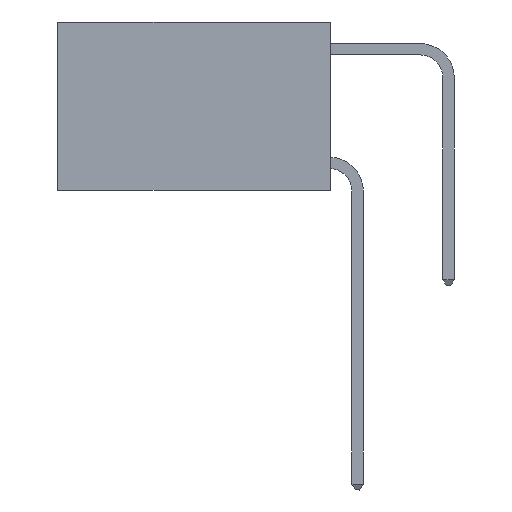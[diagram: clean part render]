
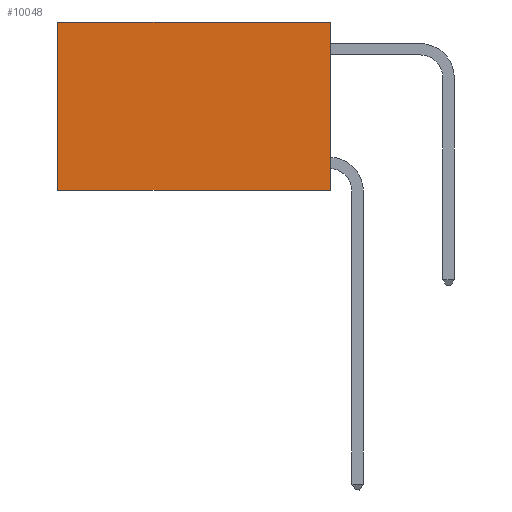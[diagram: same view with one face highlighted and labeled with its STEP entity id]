
A CAD part, left-side view. The second image highlights one B-rep face of the part: STEP entity #10048.
In plain terms, the highlighted planar face has unit normal (-1, 0, 0).
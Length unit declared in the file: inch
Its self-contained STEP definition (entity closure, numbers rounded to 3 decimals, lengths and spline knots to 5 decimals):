
#503 = PLANE ( 'NONE',  #10163 ) ;
#600 = VECTOR ( 'NONE', #11803, 39.37008 ) ;
#798 = CARTESIAN_POINT ( 'NONE',  ( 0.2625, 0.6, -0.37 ) ) ;
#1456 = DIRECTION ( 'NONE',  ( 0., 0., -1. ) ) ;
#1821 = CARTESIAN_POINT ( 'NONE',  ( 0.2625, 0., -0.37 ) ) ;
#2150 = CARTESIAN_POINT ( 'NONE',  ( 0.2625, 0.6, 0. ) ) ;
#2693 = DIRECTION ( 'NONE',  ( 0., 0., -1. ) ) ;
#3077 = EDGE_LOOP ( 'NONE', ( #4976, #9334, #11032, #4488 ) ) ;
#3455 = CARTESIAN_POINT ( 'NONE',  ( 0.2625, 0.6, 0. ) ) ;
#3558 = LINE ( 'NONE', #10167, #10643 ) ;
#3737 = CARTESIAN_POINT ( 'NONE',  ( 0.2625, 0., 0. ) ) ;
#4488 = ORIENTED_EDGE ( 'NONE', *, *, #5016, .T. ) ;
#4505 = EDGE_CURVE ( 'NONE', #13064, #6035, #13122, .T. ) ;
#4976 = ORIENTED_EDGE ( 'NONE', *, *, #4505, .T. ) ;
#5016 = EDGE_CURVE ( 'NONE', #8983, #13064, #3558, .T. ) ;
#5681 = LINE ( 'NONE', #1821, #8461 ) ;
#6035 = VERTEX_POINT ( 'NONE', #798 ) ;
#6150 = VECTOR ( 'NONE', #1456, 39.37008 ) ;
#6441 = EDGE_CURVE ( 'NONE', #8983, #9838, #9144, .T. ) ;
#7762 = CARTESIAN_POINT ( 'NONE',  ( 0.2625, 0., -0.37 ) ) ;
#8461 = VECTOR ( 'NONE', #9308, 39.37008 ) ;
#8983 = VERTEX_POINT ( 'NONE', #10709 ) ;
#9062 = DIRECTION ( 'NONE',  ( 1., 0., 0. ) ) ;
#9144 = LINE ( 'NONE', #13222, #600 ) ;
#9308 = DIRECTION ( 'NONE',  ( 0., 1., 0. ) ) ;
#9334 = ORIENTED_EDGE ( 'NONE', *, *, #12620, .F. ) ;
#9838 = VERTEX_POINT ( 'NONE', #7762 ) ;
#10048 = ADVANCED_FACE ( 'NONE', ( #12681 ), #503, .F. ) ;
#10163 = AXIS2_PLACEMENT_3D ( 'NONE', #3737, #9062, #2693 ) ;
#10167 = CARTESIAN_POINT ( 'NONE',  ( 0.2625, 0., 0. ) ) ;
#10643 = VECTOR ( 'NONE', #12005, 39.37008 ) ;
#10709 = CARTESIAN_POINT ( 'NONE',  ( 0.2625, 0., 0. ) ) ;
#11032 = ORIENTED_EDGE ( 'NONE', *, *, #6441, .F. ) ;
#11803 = DIRECTION ( 'NONE',  ( 0., 0., -1. ) ) ;
#12005 = DIRECTION ( 'NONE',  ( 0., 1., 0. ) ) ;
#12620 = EDGE_CURVE ( 'NONE', #9838, #6035, #5681, .T. ) ;
#12681 = FACE_OUTER_BOUND ( 'NONE', #3077, .T. ) ;
#13064 = VERTEX_POINT ( 'NONE', #3455 ) ;
#13122 = LINE ( 'NONE', #2150, #6150 ) ;
#13222 = CARTESIAN_POINT ( 'NONE',  ( 0.2625, 0., 0. ) ) ;
